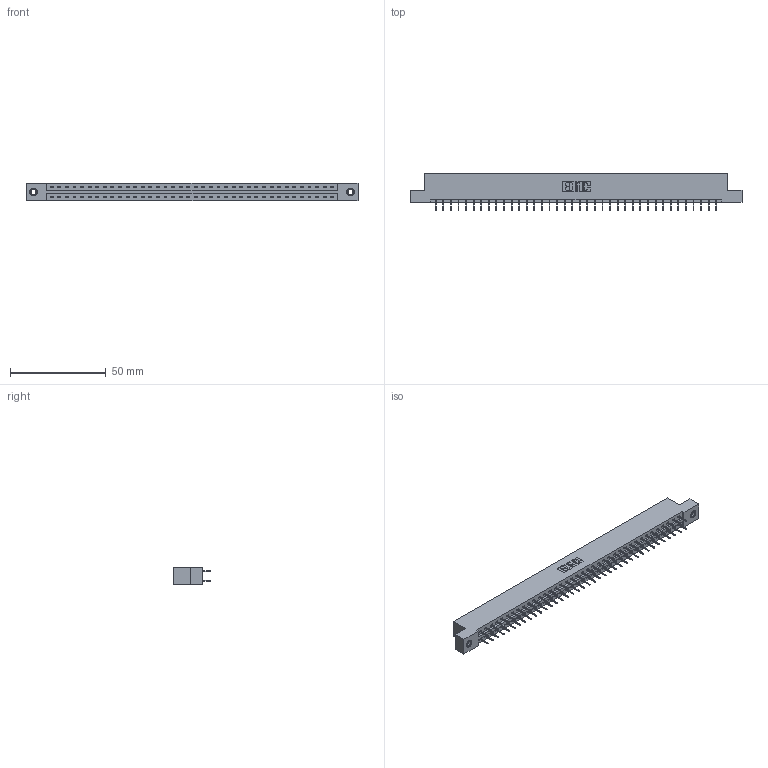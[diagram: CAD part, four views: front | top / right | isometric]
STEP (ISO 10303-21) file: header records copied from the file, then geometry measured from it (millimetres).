
FILE_DESCRIPTION (( 'STEP AP203' ), '1' );
FILE_NAME ('337-076-524-207.STEP', '2019-10-10T10:35:13', ( '' ), ( '' ), 'SwSTEP 2.0', 'SolidWorks 2016', '' );
FILE_SCHEMA (( 'CONFIG_CONTROL_DESIGN' ));
Length unit declared in the file: inch
Products named in the file (4): 345-292-001_345-293-124; 337 Part_Flush Mounting Lugs - 0.156 Dia-TI; 345-250-001_345-250-005-103; 337-076-524-207
Assembly tree (79 placements, depth 2):
  337-076-524-207
    337 Part_Flush Mounting Lugs - 0.156 Dia-TI
    345-292-001_345-293-124  x76
    345-250-001_345-250-005-103  x2
Bounding box: 173.58 x 19.69 x 9.4 mm (x, y, z)
Volume: 18111.8 mm3; surface area: 20116.4 mm2
Topology: 79 solids, 79 shells, 4582 faces, 12987 edges, 8346 vertices
Faces by surface type: plane 3446, cylinder 1120, cone 12, torus 4
Entity records: 31240 total; most frequent: CARTESIAN_POINT 5245, ORIENTED_EDGE 5174, DIRECTION 4501, EDGE_CURVE 2587, VECTOR 2443, LINE 2443, VERTEX_POINT 1716, AXIS2_PLACEMENT_3D 1029
